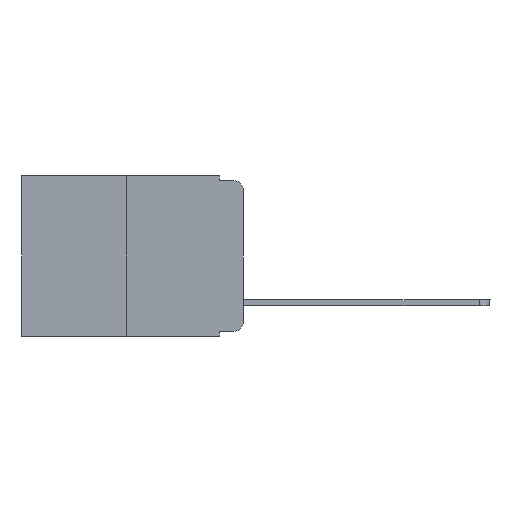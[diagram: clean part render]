
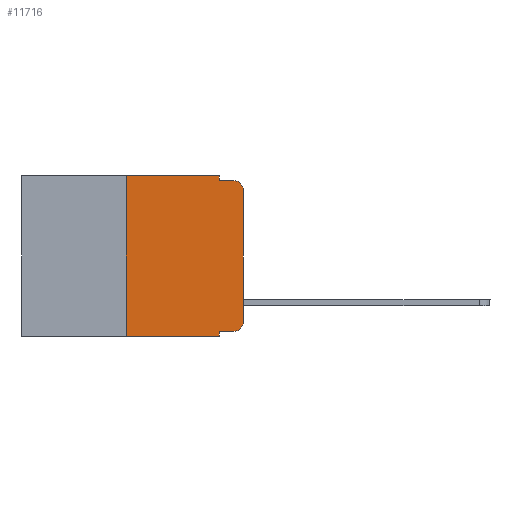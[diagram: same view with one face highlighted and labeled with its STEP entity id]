
A CAD part, left-side view. The second image highlights one B-rep face of the part: STEP entity #11716.
In plain terms, the highlighted planar face has unit normal (-1, 0, 0).
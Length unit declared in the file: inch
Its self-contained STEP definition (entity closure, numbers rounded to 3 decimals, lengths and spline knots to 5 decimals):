
#2 = VECTOR ( 'NONE', #24217, 39.37008 ) ;
#350 = FACE_OUTER_BOUND ( 'NONE', #8451, .T. ) ;
#575 = VECTOR ( 'NONE', #13274, 39.37008 ) ;
#577 = VERTEX_POINT ( 'NONE', #11454 ) ;
#979 = CARTESIAN_POINT ( 'NONE',  ( 0., 0.051, -0.333 ) ) ;
#1219 = VECTOR ( 'NONE', #10510, 39.37008 ) ;
#1322 = CARTESIAN_POINT ( 'NONE',  ( 0., 0.473, 0. ) ) ;
#1387 = CARTESIAN_POINT ( 'NONE',  ( 0., 0., -0.313 ) ) ;
#1603 = LINE ( 'NONE', #19028, #9566 ) ;
#2226 = DIRECTION ( 'NONE',  ( 0., 0., -1. ) ) ;
#2290 = CARTESIAN_POINT ( 'NONE',  ( 0., 0.25, -0.343 ) ) ;
#2561 = VERTEX_POINT ( 'NONE', #4811 ) ;
#2942 = CARTESIAN_POINT ( 'NONE',  ( 0., 0.051, 0. ) ) ;
#2994 = VERTEX_POINT ( 'NONE', #12347 ) ;
#3037 = ORIENTED_EDGE ( 'NONE', *, *, #8135, .F. ) ;
#3272 = DIRECTION ( 'NONE',  ( -1., 0., 0. ) ) ;
#3410 = ORIENTED_EDGE ( 'NONE', *, *, #8512, .F. ) ;
#4514 = ORIENTED_EDGE ( 'NONE', *, *, #13003, .T. ) ;
#4693 = ORIENTED_EDGE ( 'NONE', *, *, #12760, .T. ) ;
#4811 = CARTESIAN_POINT ( 'NONE',  ( 0., 0.051, -0.343 ) ) ;
#5231 = DIRECTION ( 'NONE',  ( 0., 0., -1. ) ) ;
#5521 = LINE ( 'NONE', #979, #16873 ) ;
#5776 = CARTESIAN_POINT ( 'NONE',  ( 0., 0.051, 0. ) ) ;
#6200 = AXIS2_PLACEMENT_3D ( 'NONE', #24914, #3272, #5231 ) ;
#7314 = VERTEX_POINT ( 'NONE', #2290 ) ;
#7839 = CARTESIAN_POINT ( 'NONE',  ( 0., 0.473, 0. ) ) ;
#7848 = CIRCLE ( 'NONE', #15066, 0.02 ) ;
#8135 = EDGE_CURVE ( 'NONE', #10900, #2994, #14119, .T. ) ;
#8451 = EDGE_LOOP ( 'NONE', ( #4693, #16812, #3037, #14999, #10754, #3410, #4514, #15933, #13577, #14578 ) ) ;
#8512 = EDGE_CURVE ( 'NONE', #7314, #11118, #11973, .T. ) ;
#8721 = CARTESIAN_POINT ( 'NONE',  ( 0., 0.473, -0.343 ) ) ;
#8834 = AXIS2_PLACEMENT_3D ( 'NONE', #7839, #21498, #2226 ) ;
#9231 = EDGE_CURVE ( 'NONE', #11118, #12550, #17426, .T. ) ;
#9566 = VECTOR ( 'NONE', #24961, 39.37008 ) ;
#10510 = DIRECTION ( 'NONE',  ( 0., -1., 0. ) ) ;
#10626 = EDGE_CURVE ( 'NONE', #577, #2561, #24750, .T. ) ;
#10754 = ORIENTED_EDGE ( 'NONE', *, *, #9231, .F. ) ;
#10900 = VERTEX_POINT ( 'NONE', #14741 ) ;
#11118 = VERTEX_POINT ( 'NONE', #15131 ) ;
#11454 = CARTESIAN_POINT ( 'NONE',  ( 0., 0.051, -0.333 ) ) ;
#11716 = ADVANCED_FACE ( 'NONE', ( #350 ), #20506, .F. ) ;
#11973 = LINE ( 'NONE', #14849, #14705 ) ;
#12259 = CARTESIAN_POINT ( 'NONE',  ( 0., 0.02, -0.313 ) ) ;
#12347 = CARTESIAN_POINT ( 'NONE',  ( 0., 0.02, -0.01 ) ) ;
#12550 = VERTEX_POINT ( 'NONE', #2942 ) ;
#12644 = EDGE_CURVE ( 'NONE', #12806, #2994, #18080, .T. ) ;
#12760 = EDGE_CURVE ( 'NONE', #21953, #12806, #12848, .T. ) ;
#12806 = VERTEX_POINT ( 'NONE', #14628 ) ;
#12848 = LINE ( 'NONE', #18522, #2 ) ;
#13003 = EDGE_CURVE ( 'NONE', #7314, #2561, #15585, .T. ) ;
#13274 = DIRECTION ( 'NONE',  ( 0., -1., 0. ) ) ;
#13577 = ORIENTED_EDGE ( 'NONE', *, *, #19438, .T. ) ;
#14119 = LINE ( 'NONE', #19984, #20583 ) ;
#14578 = ORIENTED_EDGE ( 'NONE', *, *, #15005, .T. ) ;
#14628 = CARTESIAN_POINT ( 'NONE',  ( 0., 0., -0.03 ) ) ;
#14705 = VECTOR ( 'NONE', #24491, 39.37008 ) ;
#14741 = CARTESIAN_POINT ( 'NONE',  ( 0., 0.051, -0.01 ) ) ;
#14849 = CARTESIAN_POINT ( 'NONE',  ( 0., 0.25, 0. ) ) ;
#14999 = ORIENTED_EDGE ( 'NONE', *, *, #16716, .F. ) ;
#15005 = EDGE_CURVE ( 'NONE', #23196, #21953, #7848, .T. ) ;
#15066 = AXIS2_PLACEMENT_3D ( 'NONE', #12259, #24211, #18107 ) ;
#15131 = CARTESIAN_POINT ( 'NONE',  ( 0., 0.25, 0. ) ) ;
#15585 = LINE ( 'NONE', #8721, #1219 ) ;
#15933 = ORIENTED_EDGE ( 'NONE', *, *, #10626, .F. ) ;
#16014 = DIRECTION ( 'NONE',  ( 0., -1., 0. ) ) ;
#16716 = EDGE_CURVE ( 'NONE', #12550, #10900, #1603, .T. ) ;
#16812 = ORIENTED_EDGE ( 'NONE', *, *, #12644, .T. ) ;
#16873 = VECTOR ( 'NONE', #21277, 39.37008 ) ;
#17426 = LINE ( 'NONE', #1322, #575 ) ;
#17613 = DIRECTION ( 'NONE',  ( 0., 0., -1. ) ) ;
#18080 = CIRCLE ( 'NONE', #6200, 0.02 ) ;
#18107 = DIRECTION ( 'NONE',  ( 0., 0., -1. ) ) ;
#18522 = CARTESIAN_POINT ( 'NONE',  ( 0., 0., 0. ) ) ;
#18593 = CARTESIAN_POINT ( 'NONE',  ( 0., 0.02, -0.333 ) ) ;
#19028 = CARTESIAN_POINT ( 'NONE',  ( 0., 0.051, 0. ) ) ;
#19438 = EDGE_CURVE ( 'NONE', #577, #23196, #5521, .T. ) ;
#19984 = CARTESIAN_POINT ( 'NONE',  ( 0., 0.051, -0.01 ) ) ;
#20506 = PLANE ( 'NONE',  #8834 ) ;
#20583 = VECTOR ( 'NONE', #16014, 39.37008 ) ;
#21277 = DIRECTION ( 'NONE',  ( 0., -1., 0. ) ) ;
#21498 = DIRECTION ( 'NONE',  ( 1., 0., 0. ) ) ;
#21953 = VERTEX_POINT ( 'NONE', #1387 ) ;
#23196 = VERTEX_POINT ( 'NONE', #18593 ) ;
#24151 = VECTOR ( 'NONE', #17613, 39.37008 ) ;
#24211 = DIRECTION ( 'NONE',  ( -1., 0., 0. ) ) ;
#24217 = DIRECTION ( 'NONE',  ( 0., 0., 1. ) ) ;
#24491 = DIRECTION ( 'NONE',  ( 0., 0., 1. ) ) ;
#24750 = LINE ( 'NONE', #5776, #24151 ) ;
#24914 = CARTESIAN_POINT ( 'NONE',  ( 0., 0.02, -0.03 ) ) ;
#24961 = DIRECTION ( 'NONE',  ( 0., 0., -1. ) ) ;
